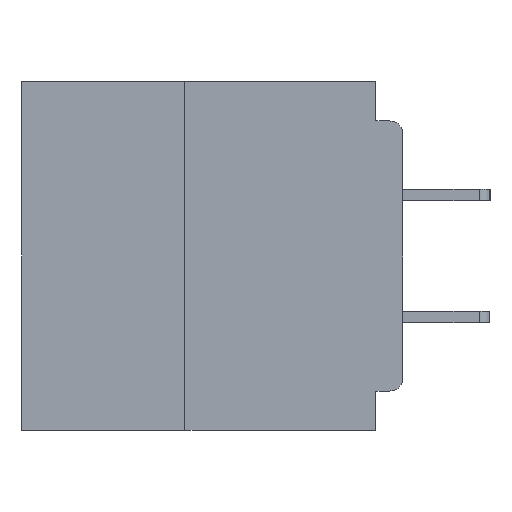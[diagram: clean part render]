
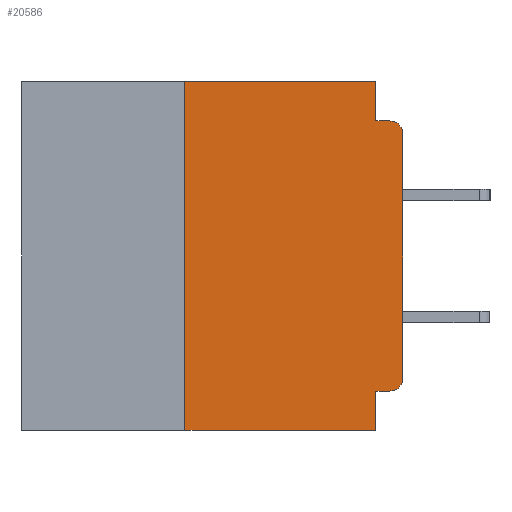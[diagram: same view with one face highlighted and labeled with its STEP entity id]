
A CAD part, left-side view. The second image highlights one B-rep face of the part: STEP entity #20586.
In plain terms, the highlighted planar face has unit normal (-1, 0, 0).
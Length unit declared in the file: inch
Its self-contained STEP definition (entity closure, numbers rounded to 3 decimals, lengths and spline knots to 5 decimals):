
#76 = LINE ( 'NONE', #25686, #32172 ) ;
#417 = FACE_OUTER_BOUND ( 'NONE', #1139, .T. ) ;
#1139 = EDGE_LOOP ( 'NONE', ( #4596, #20627, #4940, #32582, #20503, #37232, #13077, #14926, #5646, #39536 ) ) ;
#1222 = CARTESIAN_POINT ( 'NONE',  ( 0., 0.25, 0. ) ) ;
#1723 = EDGE_CURVE ( 'NONE', #23659, #3727, #30574, .T. ) ;
#1815 = EDGE_CURVE ( 'NONE', #1941, #3727, #19482, .T. ) ;
#1941 = VERTEX_POINT ( 'NONE', #3252 ) ;
#1996 = CARTESIAN_POINT ( 'NONE',  ( 0., 0.015, -0.34 ) ) ;
#2864 = CARTESIAN_POINT ( 'NONE',  ( 0., 0.015, -0.06 ) ) ;
#3252 = CARTESIAN_POINT ( 'NONE',  ( 0., 0., -0.06 ) ) ;
#3361 = CARTESIAN_POINT ( 'NONE',  ( 0., 0.25, -0.4 ) ) ;
#3727 = VERTEX_POINT ( 'NONE', #12434 ) ;
#4240 = VECTOR ( 'NONE', #4782, 39.37008 ) ;
#4440 = EDGE_CURVE ( 'NONE', #26035, #9326, #39980, .T. ) ;
#4596 = ORIENTED_EDGE ( 'NONE', *, *, #37947, .T. ) ;
#4782 = DIRECTION ( 'NONE',  ( 0., 0., 1. ) ) ;
#4916 = CARTESIAN_POINT ( 'NONE',  ( 0., 0., -0.34 ) ) ;
#4940 = ORIENTED_EDGE ( 'NONE', *, *, #1723, .F. ) ;
#5136 = DIRECTION ( 'NONE',  ( 0., 0., -1. ) ) ;
#5646 = ORIENTED_EDGE ( 'NONE', *, *, #22059, .F. ) ;
#5998 = DIRECTION ( 'NONE',  ( 0., 0., -1. ) ) ;
#6463 = VERTEX_POINT ( 'NONE', #19918 ) ;
#8340 = CIRCLE ( 'NONE', #19597, 0.015 ) ;
#9108 = CARTESIAN_POINT ( 'NONE',  ( 0., 0., -0.355 ) ) ;
#9326 = VERTEX_POINT ( 'NONE', #24955 ) ;
#11093 = VECTOR ( 'NONE', #33835, 39.37008 ) ;
#11486 = EDGE_CURVE ( 'NONE', #26035, #18217, #76, .T. ) ;
#11641 = CARTESIAN_POINT ( 'NONE',  ( 0., 0., -0.045 ) ) ;
#12434 = CARTESIAN_POINT ( 'NONE',  ( 0., 0.015, -0.045 ) ) ;
#13077 = ORIENTED_EDGE ( 'NONE', *, *, #4440, .T. ) ;
#13206 = DIRECTION ( 'NONE',  ( 0., 0., 1. ) ) ;
#14090 = CARTESIAN_POINT ( 'NONE',  ( 0., 0., 0. ) ) ;
#14117 = VECTOR ( 'NONE', #27235, 39.37008 ) ;
#14238 = EDGE_CURVE ( 'NONE', #18217, #6463, #24725, .T. ) ;
#14742 = VECTOR ( 'NONE', #35641, 39.37008 ) ;
#14926 = ORIENTED_EDGE ( 'NONE', *, *, #34106, .F. ) ;
#15208 = DIRECTION ( 'NONE',  ( 1., 0., 0. ) ) ;
#16123 = DIRECTION ( 'NONE',  ( 0., -1., 0. ) ) ;
#16347 = AXIS2_PLACEMENT_3D ( 'NONE', #2864, #24643, #5998 ) ;
#18217 = VERTEX_POINT ( 'NONE', #1222 ) ;
#18471 = VECTOR ( 'NONE', #29425, 39.37008 ) ;
#19482 = CIRCLE ( 'NONE', #16347, 0.015 ) ;
#19597 = AXIS2_PLACEMENT_3D ( 'NONE', #1996, #23790, #5136 ) ;
#19904 = LINE ( 'NONE', #14090, #4240 ) ;
#19918 = CARTESIAN_POINT ( 'NONE',  ( 0., 0.031, 0. ) ) ;
#20503 = ORIENTED_EDGE ( 'NONE', *, *, #14238, .F. ) ;
#20586 = ADVANCED_FACE ( 'NONE', ( #417 ), #24404, .F. ) ;
#20627 = ORIENTED_EDGE ( 'NONE', *, *, #1815, .T. ) ;
#21712 = VECTOR ( 'NONE', #16123, 39.37008 ) ;
#22059 = EDGE_CURVE ( 'NONE', #32510, #39685, #34733, .T. ) ;
#22433 = AXIS2_PLACEMENT_3D ( 'NONE', #33646, #15208, #36734 ) ;
#22976 = LINE ( 'NONE', #26401, #14742 ) ;
#23659 = VERTEX_POINT ( 'NONE', #29204 ) ;
#23790 = DIRECTION ( 'NONE',  ( -1., 0., 0. ) ) ;
#24404 = PLANE ( 'NONE',  #22433 ) ;
#24643 = DIRECTION ( 'NONE',  ( -1., 0., 0. ) ) ;
#24725 = LINE ( 'NONE', #38507, #18471 ) ;
#24955 = CARTESIAN_POINT ( 'NONE',  ( 0., 0.031, -0.4 ) ) ;
#25312 = DIRECTION ( 'NONE',  ( 0., 0., -1. ) ) ;
#25538 = CARTESIAN_POINT ( 'NONE',  ( 0., 0.031, -0.355 ) ) ;
#25686 = CARTESIAN_POINT ( 'NONE',  ( 0., 0.25, -0.4 ) ) ;
#26035 = VERTEX_POINT ( 'NONE', #3361 ) ;
#26401 = CARTESIAN_POINT ( 'NONE',  ( 0., 0.031, 0. ) ) ;
#27235 = DIRECTION ( 'NONE',  ( 0., -1., 0. ) ) ;
#27804 = CARTESIAN_POINT ( 'NONE',  ( 0., 0.015, -0.355 ) ) ;
#29204 = CARTESIAN_POINT ( 'NONE',  ( 0., 0.031, -0.045 ) ) ;
#29425 = DIRECTION ( 'NONE',  ( 0., -1., 0. ) ) ;
#30242 = VERTEX_POINT ( 'NONE', #4916 ) ;
#30574 = LINE ( 'NONE', #11641, #14117 ) ;
#31458 = CARTESIAN_POINT ( 'NONE',  ( 0., 0.437, -0.4 ) ) ;
#32169 = VECTOR ( 'NONE', #25312, 39.37008 ) ;
#32172 = VECTOR ( 'NONE', #13206, 39.37008 ) ;
#32510 = VERTEX_POINT ( 'NONE', #27804 ) ;
#32582 = ORIENTED_EDGE ( 'NONE', *, *, #35653, .F. ) ;
#33646 = CARTESIAN_POINT ( 'NONE',  ( 0., 0.437, 0. ) ) ;
#33835 = DIRECTION ( 'NONE',  ( 0., 1., 0. ) ) ;
#34106 = EDGE_CURVE ( 'NONE', #39685, #9326, #39389, .T. ) ;
#34378 = CARTESIAN_POINT ( 'NONE',  ( 0., 0.031, -0.4 ) ) ;
#34733 = LINE ( 'NONE', #9108, #11093 ) ;
#35641 = DIRECTION ( 'NONE',  ( 0., 0., -1. ) ) ;
#35653 = EDGE_CURVE ( 'NONE', #6463, #23659, #22976, .T. ) ;
#36734 = DIRECTION ( 'NONE',  ( 0., 0., -1. ) ) ;
#37232 = ORIENTED_EDGE ( 'NONE', *, *, #11486, .F. ) ;
#37947 = EDGE_CURVE ( 'NONE', #30242, #1941, #19904, .T. ) ;
#38507 = CARTESIAN_POINT ( 'NONE',  ( 0., 0.437, 0. ) ) ;
#38596 = EDGE_CURVE ( 'NONE', #32510, #30242, #8340, .T. ) ;
#39389 = LINE ( 'NONE', #34378, #32169 ) ;
#39536 = ORIENTED_EDGE ( 'NONE', *, *, #38596, .T. ) ;
#39685 = VERTEX_POINT ( 'NONE', #25538 ) ;
#39980 = LINE ( 'NONE', #31458, #21712 ) ;
